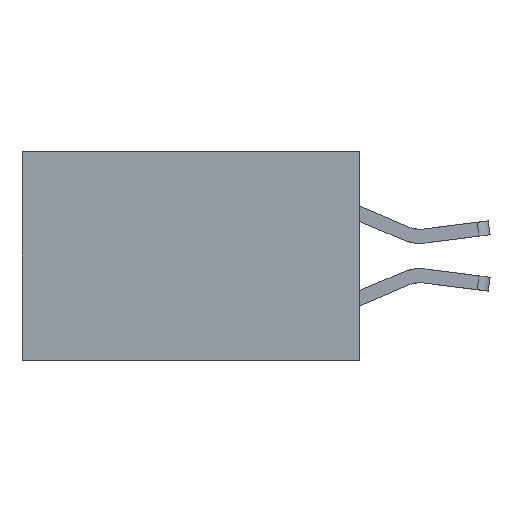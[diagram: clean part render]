
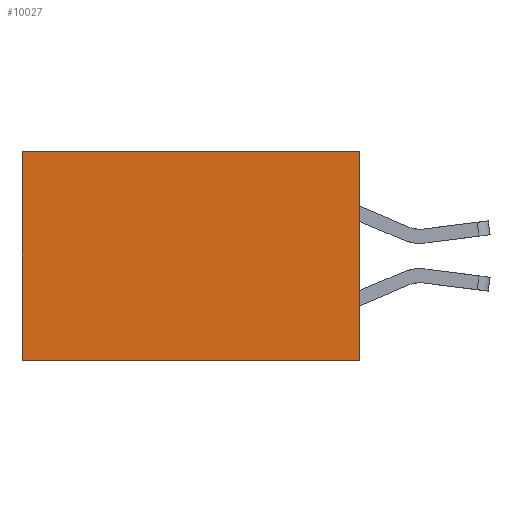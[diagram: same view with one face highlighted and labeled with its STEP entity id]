
A CAD part, left-side view. The second image highlights one B-rep face of the part: STEP entity #10027.
In plain terms, the highlighted planar face has unit normal (-1, 0, 0).
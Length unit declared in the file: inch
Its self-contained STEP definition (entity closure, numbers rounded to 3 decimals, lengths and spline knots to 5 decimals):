
#21 = CARTESIAN_POINT ( 'NONE',  ( 0.2875, 0., 0. ) ) ;
#251 = EDGE_LOOP ( 'NONE', ( #7043, #408, #8683, #16520 ) ) ;
#408 = ORIENTED_EDGE ( 'NONE', *, *, #12605, .F. ) ;
#527 = EDGE_CURVE ( 'NONE', #9436, #12159, #875, .T. ) ;
#875 = LINE ( 'NONE', #21, #16371 ) ;
#1808 = CARTESIAN_POINT ( 'NONE',  ( 0.2875, 0.6, 0. ) ) ;
#2270 = VERTEX_POINT ( 'NONE', #8031 ) ;
#2361 = PLANE ( 'NONE',  #14072 ) ;
#2888 = DIRECTION ( 'NONE',  ( 0., 1., 0. ) ) ;
#3439 = DIRECTION ( 'NONE',  ( 0., 0., -1. ) ) ;
#3472 = CARTESIAN_POINT ( 'NONE',  ( 0.2875, 0., -0.37 ) ) ;
#3719 = LINE ( 'NONE', #15813, #17274 ) ;
#4093 = CARTESIAN_POINT ( 'NONE',  ( 0.2875, 0., -0.37 ) ) ;
#4488 = LINE ( 'NONE', #5759, #17178 ) ;
#5759 = CARTESIAN_POINT ( 'NONE',  ( 0.2875, 0., 0. ) ) ;
#6631 = CARTESIAN_POINT ( 'NONE',  ( 0.2875, 0., 0. ) ) ;
#6997 = CARTESIAN_POINT ( 'NONE',  ( 0.2875, 0., 0. ) ) ;
#7043 = ORIENTED_EDGE ( 'NONE', *, *, #17937, .T. ) ;
#7739 = LINE ( 'NONE', #3472, #14298 ) ;
#8031 = CARTESIAN_POINT ( 'NONE',  ( 0.2875, 0.6, -0.37 ) ) ;
#8683 = ORIENTED_EDGE ( 'NONE', *, *, #527, .F. ) ;
#9436 = VERTEX_POINT ( 'NONE', #6997 ) ;
#10027 = ADVANCED_FACE ( 'NONE', ( #17865 ), #2361, .F. ) ;
#10851 = DIRECTION ( 'NONE',  ( 1., 0., 0. ) ) ;
#12159 = VERTEX_POINT ( 'NONE', #4093 ) ;
#12605 = EDGE_CURVE ( 'NONE', #12159, #2270, #7739, .T. ) ;
#12885 = EDGE_CURVE ( 'NONE', #9436, #16558, #4488, .T. ) ;
#14072 = AXIS2_PLACEMENT_3D ( 'NONE', #6631, #10851, #17656 ) ;
#14298 = VECTOR ( 'NONE', #17648, 39.37008 ) ;
#15813 = CARTESIAN_POINT ( 'NONE',  ( 0.2875, 0.6, 0. ) ) ;
#16371 = VECTOR ( 'NONE', #16787, 39.37008 ) ;
#16520 = ORIENTED_EDGE ( 'NONE', *, *, #12885, .T. ) ;
#16558 = VERTEX_POINT ( 'NONE', #1808 ) ;
#16787 = DIRECTION ( 'NONE',  ( 0., 0., -1. ) ) ;
#17178 = VECTOR ( 'NONE', #2888, 39.37008 ) ;
#17274 = VECTOR ( 'NONE', #3439, 39.37008 ) ;
#17648 = DIRECTION ( 'NONE',  ( 0., 1., 0. ) ) ;
#17656 = DIRECTION ( 'NONE',  ( 0., 0., -1. ) ) ;
#17865 = FACE_OUTER_BOUND ( 'NONE', #251, .T. ) ;
#17937 = EDGE_CURVE ( 'NONE', #16558, #2270, #3719, .T. ) ;
